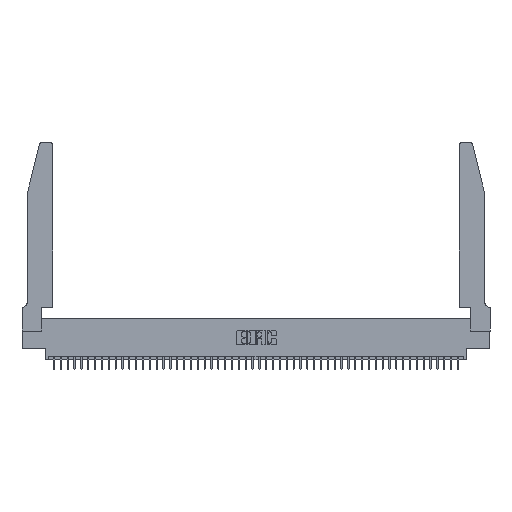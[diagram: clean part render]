
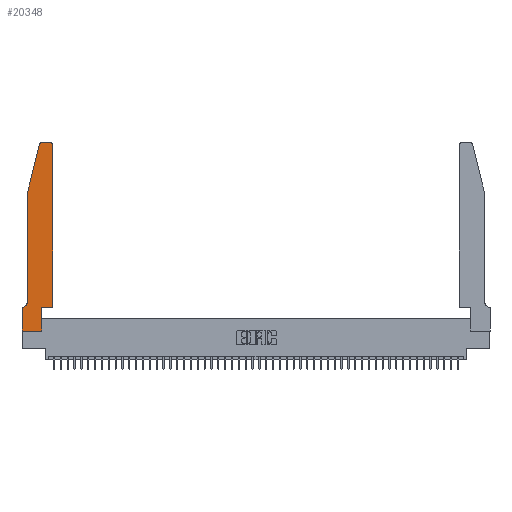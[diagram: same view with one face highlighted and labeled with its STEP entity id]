
A CAD part, top view. The second image highlights one B-rep face of the part: STEP entity #20348.
In plain terms, the highlighted planar face has unit normal (0, 0, 1).
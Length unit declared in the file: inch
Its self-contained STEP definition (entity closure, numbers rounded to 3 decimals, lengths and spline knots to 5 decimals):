
#579 = AXIS2_PLACEMENT_3D ( 'NONE', #1545, #40013, #17164 ) ;
#984 = EDGE_LOOP ( 'NONE', ( #44529, #20138, #30208, #46980, #5346, #1531, #7173, #5001, #11754, #43696, #48477, #48108 ) ) ;
#1307 = EDGE_CURVE ( 'NONE', #6661, #1609, #8460, .T. ) ;
#1443 = CARTESIAN_POINT ( 'NONE',  ( 0.2605, 2.75, 0.37 ) ) ;
#1531 = ORIENTED_EDGE ( 'NONE', *, *, #1307, .T. ) ;
#1545 = CARTESIAN_POINT ( 'NONE',  ( 0.4205, 2.72, 0.37 ) ) ;
#1609 = VERTEX_POINT ( 'NONE', #47505 ) ;
#1788 = EDGE_CURVE ( 'NONE', #23462, #6661, #40975, .T. ) ;
#2350 = VECTOR ( 'NONE', #36964, 39.37008 ) ;
#3014 = CARTESIAN_POINT ( 'NONE',  ( 0.4505, 0.35, 0.37 ) ) ;
#3943 = CARTESIAN_POINT ( 'NONE',  ( 0.2865, 0., 0.37 ) ) ;
#5001 = ORIENTED_EDGE ( 'NONE', *, *, #29088, .T. ) ;
#5346 = ORIENTED_EDGE ( 'NONE', *, *, #1788, .T. ) ;
#5421 = CARTESIAN_POINT ( 'NONE',  ( 0.0755, 2., 0.37 ) ) ;
#5818 = DIRECTION ( 'NONE',  ( 0., 0., -1. ) ) ;
#6381 = DIRECTION ( 'NONE',  ( 0., 0., 1. ) ) ;
#6407 = LINE ( 'NONE', #30295, #40281 ) ;
#6661 = VERTEX_POINT ( 'NONE', #45042 ) ;
#7133 = CIRCLE ( 'NONE', #45653, 0.03 ) ;
#7173 = ORIENTED_EDGE ( 'NONE', *, *, #45667, .T. ) ;
#7350 = CARTESIAN_POINT ( 'NONE',  ( 0.2865, 0.35, 0.37 ) ) ;
#8460 = LINE ( 'NONE', #12492, #30528 ) ;
#8684 = CARTESIAN_POINT ( 'NONE',  ( 0.2865, 0.35, 0.37 ) ) ;
#9932 = LINE ( 'NONE', #5421, #20066 ) ;
#10061 = CARTESIAN_POINT ( 'NONE',  ( 0.4505, 0.35, 0.37 ) ) ;
#10072 = CARTESIAN_POINT ( 'NONE',  ( 0.4505, 0.35, 0.37 ) ) ;
#10398 = DIRECTION ( 'NONE',  ( 1., 0., 0. ) ) ;
#11754 = ORIENTED_EDGE ( 'NONE', *, *, #24425, .T. ) ;
#12492 = CARTESIAN_POINT ( 'NONE',  ( 0.0755, 0.35, 0.37 ) ) ;
#13092 = CARTESIAN_POINT ( 'NONE',  ( 0.4205, 2.75, 0.37 ) ) ;
#13939 = CARTESIAN_POINT ( 'NONE',  ( 0., 0.35, 0.37 ) ) ;
#14379 = DIRECTION ( 'NONE',  ( -1., 0., 0. ) ) ;
#15189 = CARTESIAN_POINT ( 'NONE',  ( 0.0755, 0.42, 0.37 ) ) ;
#15428 = VECTOR ( 'NONE', #43547, 39.37008 ) ;
#15658 = EDGE_CURVE ( 'NONE', #32246, #18716, #7133, .T. ) ;
#16448 = EDGE_CURVE ( 'NONE', #17242, #35555, #25651, .T. ) ;
#16461 = CARTESIAN_POINT ( 'NONE',  ( 0., 0., 0.37 ) ) ;
#16672 = CARTESIAN_POINT ( 'NONE',  ( 0.0755, 2., 0.37 ) ) ;
#17164 = DIRECTION ( 'NONE',  ( 1., 0., 0. ) ) ;
#17242 = VERTEX_POINT ( 'NONE', #7350 ) ;
#17250 = DIRECTION ( 'NONE',  ( -0.239, -0.971, 0. ) ) ;
#18165 = VERTEX_POINT ( 'NONE', #23322 ) ;
#18249 = CARTESIAN_POINT ( 'NONE',  ( 0.284, 2.75, 0.37 ) ) ;
#18716 = VERTEX_POINT ( 'NONE', #27276 ) ;
#19157 = CARTESIAN_POINT ( 'NONE',  ( 0., 0., 0.37 ) ) ;
#19297 = VECTOR ( 'NONE', #46628, 39.37008 ) ;
#19412 = VECTOR ( 'NONE', #28118, 39.37008 ) ;
#20066 = VECTOR ( 'NONE', #17250, 39.37008 ) ;
#20138 = ORIENTED_EDGE ( 'NONE', *, *, #15658, .T. ) ;
#20348 = ADVANCED_FACE ( 'NONE', ( #48592 ), #37060, .T. ) ;
#20452 = LINE ( 'NONE', #16672, #15428 ) ;
#23322 = CARTESIAN_POINT ( 'NONE',  ( 0.4505, 2.72, 0.37 ) ) ;
#23462 = VERTEX_POINT ( 'NONE', #15189 ) ;
#24007 = CARTESIAN_POINT ( 'NONE',  ( 0.0755, 2., 0.37 ) ) ;
#24425 = EDGE_CURVE ( 'NONE', #31716, #17242, #31099, .T. ) ;
#24515 = DIRECTION ( 'NONE',  ( 0., 0., 1. ) ) ;
#24536 = EDGE_CURVE ( 'NONE', #18716, #36564, #9932, .T. ) ;
#25651 = LINE ( 'NONE', #3014, #2350 ) ;
#27276 = CARTESIAN_POINT ( 'NONE',  ( 0.25487, 2.72718, 0.37 ) ) ;
#28118 = DIRECTION ( 'NONE',  ( -1., 0., 0. ) ) ;
#28332 = DIRECTION ( 'NONE',  ( -1., 0., 0. ) ) ;
#29088 = EDGE_CURVE ( 'NONE', #36553, #31716, #6407, .T. ) ;
#29326 = EDGE_CURVE ( 'NONE', #36564, #23462, #20452, .T. ) ;
#30208 = ORIENTED_EDGE ( 'NONE', *, *, #24536, .T. ) ;
#30295 = CARTESIAN_POINT ( 'NONE',  ( 0., 0., 0.37 ) ) ;
#30528 = VECTOR ( 'NONE', #28332, 39.37008 ) ;
#31099 = LINE ( 'NONE', #8684, #19297 ) ;
#31716 = VERTEX_POINT ( 'NONE', #3943 ) ;
#32246 = VERTEX_POINT ( 'NONE', #18249 ) ;
#32371 = VERTEX_POINT ( 'NONE', #13092 ) ;
#34230 = DIRECTION ( 'NONE',  ( 0., -1., 0. ) ) ;
#35555 = VERTEX_POINT ( 'NONE', #10072 ) ;
#35913 = CIRCLE ( 'NONE', #579, 0.03 ) ;
#36553 = VERTEX_POINT ( 'NONE', #16461 ) ;
#36564 = VERTEX_POINT ( 'NONE', #24007 ) ;
#36964 = DIRECTION ( 'NONE',  ( 1., 0., 0. ) ) ;
#37026 = EDGE_CURVE ( 'NONE', #18165, #32371, #35913, .T. ) ;
#37060 = PLANE ( 'NONE',  #37138 ) ;
#37138 = AXIS2_PLACEMENT_3D ( 'NONE', #13939, #6381, #10398 ) ;
#40013 = DIRECTION ( 'NONE',  ( 0., 0., 1. ) ) ;
#40281 = VECTOR ( 'NONE', #45105, 39.37008 ) ;
#40594 = EDGE_CURVE ( 'NONE', #32371, #32246, #47420, .T. ) ;
#40975 = CIRCLE ( 'NONE', #44172, 0.07 ) ;
#42006 = LINE ( 'NONE', #19157, #45281 ) ;
#43341 = CARTESIAN_POINT ( 'NONE',  ( 0.284, 2.72, 0.37 ) ) ;
#43547 = DIRECTION ( 'NONE',  ( 0., -1., 0. ) ) ;
#43696 = ORIENTED_EDGE ( 'NONE', *, *, #16448, .T. ) ;
#44172 = AXIS2_PLACEMENT_3D ( 'NONE', #48262, #5818, #14379 ) ;
#44429 = VECTOR ( 'NONE', #44757, 39.37008 ) ;
#44529 = ORIENTED_EDGE ( 'NONE', *, *, #40594, .T. ) ;
#44757 = DIRECTION ( 'NONE',  ( 0., 1., 0. ) ) ;
#44967 = EDGE_CURVE ( 'NONE', #35555, #18165, #47747, .T. ) ;
#45042 = CARTESIAN_POINT ( 'NONE',  ( 0.0055, 0.35, 0.37 ) ) ;
#45105 = DIRECTION ( 'NONE',  ( 1., 0., 0. ) ) ;
#45281 = VECTOR ( 'NONE', #34230, 39.37008 ) ;
#45653 = AXIS2_PLACEMENT_3D ( 'NONE', #43341, #24515, #47334 ) ;
#45667 = EDGE_CURVE ( 'NONE', #1609, #36553, #42006, .T. ) ;
#46628 = DIRECTION ( 'NONE',  ( 0., 1., 0. ) ) ;
#46980 = ORIENTED_EDGE ( 'NONE', *, *, #29326, .T. ) ;
#47334 = DIRECTION ( 'NONE',  ( 1., 0., 0. ) ) ;
#47420 = LINE ( 'NONE', #1443, #19412 ) ;
#47505 = CARTESIAN_POINT ( 'NONE',  ( 0., 0.35, 0.37 ) ) ;
#47747 = LINE ( 'NONE', #10061, #44429 ) ;
#48108 = ORIENTED_EDGE ( 'NONE', *, *, #37026, .T. ) ;
#48262 = CARTESIAN_POINT ( 'NONE',  ( 0.0055, 0.42, 0.37 ) ) ;
#48477 = ORIENTED_EDGE ( 'NONE', *, *, #44967, .T. ) ;
#48592 = FACE_OUTER_BOUND ( 'NONE', #984, .T. ) ;
